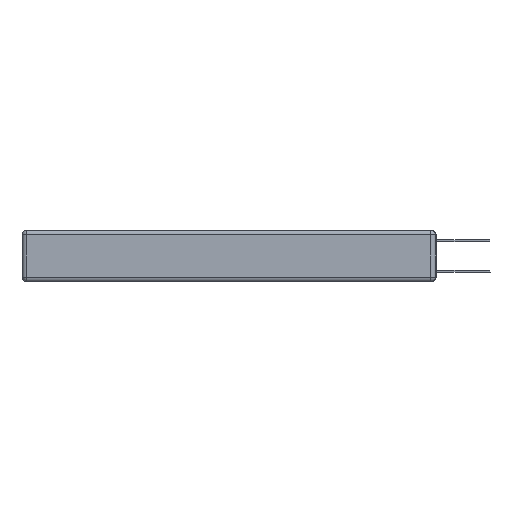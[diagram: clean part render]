
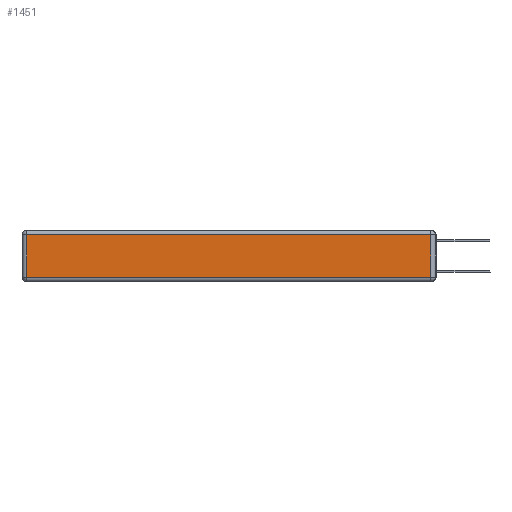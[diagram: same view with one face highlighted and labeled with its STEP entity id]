
A CAD part, left-side view. The second image highlights one B-rep face of the part: STEP entity #1451.
In plain terms, the highlighted planar face has unit normal (-1, 0, 0).
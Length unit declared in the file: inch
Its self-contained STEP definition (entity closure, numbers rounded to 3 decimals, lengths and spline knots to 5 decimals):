
#73 = VERTEX_POINT ( 'NONE', #6222 ) ;
#415 = EDGE_CURVE ( 'NONE', #19254, #3640, #24597, .T. ) ;
#1361 = CARTESIAN_POINT ( 'NONE',  ( 0., 0.03, -0.313 ) ) ;
#1451 = ADVANCED_FACE ( 'NONE', ( #3628 ), #23045, .T. ) ;
#2018 = CARTESIAN_POINT ( 'NONE',  ( 0., 2.75, -0.03 ) ) ;
#2176 = EDGE_CURVE ( 'NONE', #73, #19254, #11378, .T. ) ;
#2239 = VERTEX_POINT ( 'NONE', #16294 ) ;
#3040 = DIRECTION ( 'NONE',  ( 0., -1., 0. ) ) ;
#3279 = VECTOR ( 'NONE', #3040, 39.37008 ) ;
#3628 = FACE_OUTER_BOUND ( 'NONE', #9665, .T. ) ;
#3640 = VERTEX_POINT ( 'NONE', #19220 ) ;
#3657 = EDGE_CURVE ( 'NONE', #3640, #2239, #21980, .T. ) ;
#4545 = DIRECTION ( 'NONE',  ( 0., 0., -1. ) ) ;
#6222 = CARTESIAN_POINT ( 'NONE',  ( 0., 2.72, -0.313 ) ) ;
#6788 = VECTOR ( 'NONE', #15367, 39.37008 ) ;
#7945 = DIRECTION ( 'NONE',  ( 0., 0., 1. ) ) ;
#8147 = CARTESIAN_POINT ( 'NONE',  ( 0., 2.72, -0.343 ) ) ;
#9665 = EDGE_LOOP ( 'NONE', ( #10615, #14246, #20991, #11467 ) ) ;
#10615 = ORIENTED_EDGE ( 'NONE', *, *, #2176, .T. ) ;
#11378 = LINE ( 'NONE', #12588, #3279 ) ;
#11467 = ORIENTED_EDGE ( 'NONE', *, *, #12441, .T. ) ;
#11908 = DIRECTION ( 'NONE',  ( 0., 0., 1. ) ) ;
#12441 = EDGE_CURVE ( 'NONE', #2239, #73, #18186, .T. ) ;
#12588 = CARTESIAN_POINT ( 'NONE',  ( 0., 0., -0.313 ) ) ;
#14246 = ORIENTED_EDGE ( 'NONE', *, *, #415, .T. ) ;
#15367 = DIRECTION ( 'NONE',  ( 0., 1., 0. ) ) ;
#15569 = DIRECTION ( 'NONE',  ( -1., 0., 0. ) ) ;
#16294 = CARTESIAN_POINT ( 'NONE',  ( 0., 2.72, -0.03 ) ) ;
#18049 = AXIS2_PLACEMENT_3D ( 'NONE', #21336, #15569, #7945 ) ;
#18186 = LINE ( 'NONE', #8147, #21179 ) ;
#19220 = CARTESIAN_POINT ( 'NONE',  ( 0., 0.03, -0.03 ) ) ;
#19254 = VERTEX_POINT ( 'NONE', #1361 ) ;
#20943 = CARTESIAN_POINT ( 'NONE',  ( 0., 0.03, -0.343 ) ) ;
#20991 = ORIENTED_EDGE ( 'NONE', *, *, #3657, .T. ) ;
#21179 = VECTOR ( 'NONE', #4545, 39.37008 ) ;
#21336 = CARTESIAN_POINT ( 'NONE',  ( 0., 0., -0.343 ) ) ;
#21980 = LINE ( 'NONE', #2018, #6788 ) ;
#22471 = VECTOR ( 'NONE', #11908, 39.37008 ) ;
#23045 = PLANE ( 'NONE',  #18049 ) ;
#24597 = LINE ( 'NONE', #20943, #22471 ) ;
